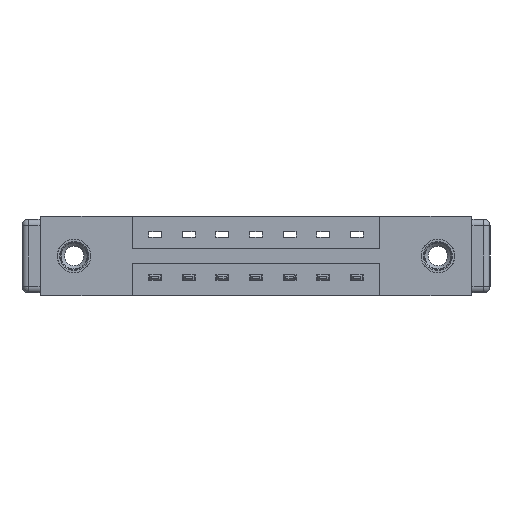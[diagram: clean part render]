
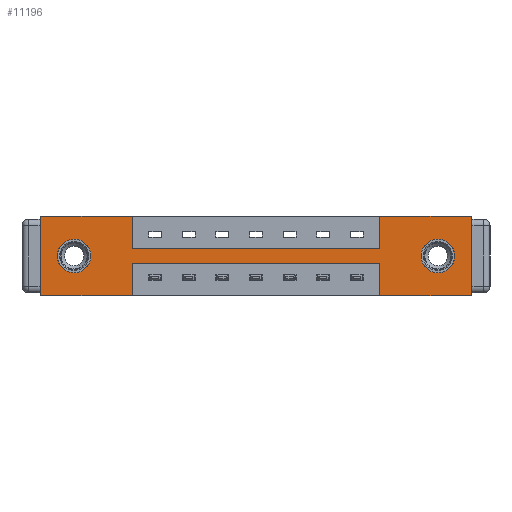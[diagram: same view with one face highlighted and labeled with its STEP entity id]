
A CAD part, front view. The second image highlights one B-rep face of the part: STEP entity #11196.
In plain terms, the highlighted planar face has unit normal (0, -1, 0).
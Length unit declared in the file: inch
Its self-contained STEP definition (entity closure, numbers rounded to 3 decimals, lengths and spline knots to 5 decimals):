
#67 = LINE ( 'NONE', #10866, #672 ) ;
#91 = EDGE_CURVE ( 'NONE', #1367, #12182, #2220, .T. ) ;
#122 = CARTESIAN_POINT ( 'NONE',  ( 0.425, 0., 0. ) ) ;
#201 = LINE ( 'NONE', #8902, #2409 ) ;
#452 = VECTOR ( 'NONE', #4776, 39.37008 ) ;
#585 = EDGE_LOOP ( 'NONE', ( #9365, #6233 ) ) ;
#595 = VERTEX_POINT ( 'NONE', #9121 ) ;
#672 = VECTOR ( 'NONE', #8072, 39.37008 ) ;
#810 = EDGE_CURVE ( 'NONE', #12182, #1367, #10688, .T. ) ;
#855 = ORIENTED_EDGE ( 'NONE', *, *, #3293, .F. ) ;
#969 = EDGE_CURVE ( 'NONE', #11671, #3734, #5891, .T. ) ;
#1114 = CARTESIAN_POINT ( 'NONE',  ( 0., 0., -0.37 ) ) ;
#1260 = CARTESIAN_POINT ( 'NONE',  ( 0., 0., -0.37 ) ) ;
#1367 = VERTEX_POINT ( 'NONE', #10426 ) ;
#1386 = LINE ( 'NONE', #1260, #7790 ) ;
#1478 = LINE ( 'NONE', #8052, #5311 ) ;
#1542 = AXIS2_PLACEMENT_3D ( 'NONE', #10679, #2914, #8666 ) ;
#1569 = VERTEX_POINT ( 'NONE', #11350 ) ;
#1675 = CARTESIAN_POINT ( 'NONE',  ( 0.425, 0., -0.15 ) ) ;
#1764 = CARTESIAN_POINT ( 'NONE',  ( 0.425, 0., -0.22 ) ) ;
#1878 = ORIENTED_EDGE ( 'NONE', *, *, #9618, .F. ) ;
#1949 = VECTOR ( 'NONE', #7408, 39.37008 ) ;
#2204 = CIRCLE ( 'NONE', #6351, 0.078 ) ;
#2214 = VECTOR ( 'NONE', #3540, 39.37008 ) ;
#2220 = CIRCLE ( 'NONE', #11262, 0.078 ) ;
#2244 = CARTESIAN_POINT ( 'NONE',  ( 1.843, 0., -0.185 ) ) ;
#2322 = CARTESIAN_POINT ( 'NONE',  ( 1.843, 0., -0.185 ) ) ;
#2409 = VECTOR ( 'NONE', #6393, 39.37008 ) ;
#2914 = DIRECTION ( 'NONE',  ( 0., 1., 0. ) ) ;
#3177 = ORIENTED_EDGE ( 'NONE', *, *, #4424, .T. ) ;
#3228 = DIRECTION ( 'NONE',  ( 0., 1., 0. ) ) ;
#3293 = EDGE_CURVE ( 'NONE', #7916, #9405, #5534, .T. ) ;
#3355 = CARTESIAN_POINT ( 'NONE',  ( 0.425, 0., -0.15 ) ) ;
#3430 = ORIENTED_EDGE ( 'NONE', *, *, #3432, .F. ) ;
#3432 = EDGE_CURVE ( 'NONE', #12314, #11671, #67, .T. ) ;
#3437 = EDGE_LOOP ( 'NONE', ( #6047, #3430, #1878, #6123, #7383, #6937, #9021, #7104, #6111, #855, #9856, #11272 ) ) ;
#3540 = DIRECTION ( 'NONE',  ( 0., 0., -1. ) ) ;
#3650 = CARTESIAN_POINT ( 'NONE',  ( 1.843, 0., -0.263 ) ) ;
#3734 = VERTEX_POINT ( 'NONE', #6125 ) ;
#3785 = AXIS2_PLACEMENT_3D ( 'NONE', #8471, #11432, #6671 ) ;
#3969 = DIRECTION ( 'NONE',  ( 0., 1., 0. ) ) ;
#4102 = CARTESIAN_POINT ( 'NONE',  ( 0.155, 0., -0.185 ) ) ;
#4159 = EDGE_CURVE ( 'NONE', #3734, #11264, #1386, .T. ) ;
#4201 = EDGE_CURVE ( 'NONE', #7337, #9529, #10927, .T. ) ;
#4424 = EDGE_CURVE ( 'NONE', #5752, #9320, #11345, .T. ) ;
#4460 = EDGE_CURVE ( 'NONE', #9405, #7337, #5518, .T. ) ;
#4485 = DIRECTION ( 'NONE',  ( 0., 0., -1. ) ) ;
#4542 = EDGE_LOOP ( 'NONE', ( #3177, #9253 ) ) ;
#4626 = VECTOR ( 'NONE', #12281, 39.37008 ) ;
#4670 = CARTESIAN_POINT ( 'NONE',  ( 1.573, 0., -0.37 ) ) ;
#4697 = CARTESIAN_POINT ( 'NONE',  ( 1.573, 0., 0. ) ) ;
#4776 = DIRECTION ( 'NONE',  ( 1., 0., 0. ) ) ;
#4903 = VECTOR ( 'NONE', #7796, 39.37008 ) ;
#5211 = DIRECTION ( 'NONE',  ( 0., 0., 1. ) ) ;
#5311 = VECTOR ( 'NONE', #5211, 39.37008 ) ;
#5518 = LINE ( 'NONE', #6795, #10326 ) ;
#5534 = LINE ( 'NONE', #9339, #4626 ) ;
#5566 = EDGE_CURVE ( 'NONE', #9529, #9190, #10666, .T. ) ;
#5608 = LINE ( 'NONE', #10615, #452 ) ;
#5752 = VERTEX_POINT ( 'NONE', #6143 ) ;
#5885 = DIRECTION ( 'NONE',  ( -1., 0., 0. ) ) ;
#5891 = LINE ( 'NONE', #10244, #7719 ) ;
#6019 = DIRECTION ( 'NONE',  ( 0., 0., 1. ) ) ;
#6047 = ORIENTED_EDGE ( 'NONE', *, *, #969, .F. ) ;
#6055 = DIRECTION ( 'NONE',  ( 0., 0., -1. ) ) ;
#6085 = DIRECTION ( 'NONE',  ( 0., 0., -1. ) ) ;
#6111 = ORIENTED_EDGE ( 'NONE', *, *, #4460, .F. ) ;
#6123 = ORIENTED_EDGE ( 'NONE', *, *, #7729, .F. ) ;
#6125 = CARTESIAN_POINT ( 'NONE',  ( 0.425, 0., -0.37 ) ) ;
#6143 = CARTESIAN_POINT ( 'NONE',  ( 1.843, 0., -0.107 ) ) ;
#6233 = ORIENTED_EDGE ( 'NONE', *, *, #810, .T. ) ;
#6351 = AXIS2_PLACEMENT_3D ( 'NONE', #2244, #3228, #6055 ) ;
#6393 = DIRECTION ( 'NONE',  ( -1., 0., 0. ) ) ;
#6636 = FACE_OUTER_BOUND ( 'NONE', #3437, .T. ) ;
#6671 = DIRECTION ( 'NONE',  ( 0., 0., -1. ) ) ;
#6795 = CARTESIAN_POINT ( 'NONE',  ( 0.425, 0., 0. ) ) ;
#6877 = LINE ( 'NONE', #10425, #1949 ) ;
#6937 = ORIENTED_EDGE ( 'NONE', *, *, #10081, .F. ) ;
#7065 = AXIS2_PLACEMENT_3D ( 'NONE', #2322, #10871, #6085 ) ;
#7104 = ORIENTED_EDGE ( 'NONE', *, *, #4201, .F. ) ;
#7236 = FACE_BOUND ( 'NONE', #585, .T. ) ;
#7265 = LINE ( 'NONE', #7524, #2214 ) ;
#7337 = VERTEX_POINT ( 'NONE', #1675 ) ;
#7383 = ORIENTED_EDGE ( 'NONE', *, *, #9859, .F. ) ;
#7403 = EDGE_CURVE ( 'NONE', #11264, #7916, #6877, .T. ) ;
#7407 = VERTEX_POINT ( 'NONE', #4670 ) ;
#7408 = DIRECTION ( 'NONE',  ( 0., 0., 1. ) ) ;
#7478 = PLANE ( 'NONE',  #3785 ) ;
#7524 = CARTESIAN_POINT ( 'NONE',  ( 1.998, 0., 0. ) ) ;
#7719 = VECTOR ( 'NONE', #4485, 39.37008 ) ;
#7729 = EDGE_CURVE ( 'NONE', #595, #7407, #201, .T. ) ;
#7790 = VECTOR ( 'NONE', #5885, 39.37008 ) ;
#7796 = DIRECTION ( 'NONE',  ( 1., 0., 0. ) ) ;
#7916 = VERTEX_POINT ( 'NONE', #10292 ) ;
#8052 = CARTESIAN_POINT ( 'NONE',  ( 1.573, 0., -0.37 ) ) ;
#8072 = DIRECTION ( 'NONE',  ( -1., 0., 0. ) ) ;
#8147 = VECTOR ( 'NONE', #11400, 39.37008 ) ;
#8274 = CARTESIAN_POINT ( 'NONE',  ( 1.573, 0., 0. ) ) ;
#8471 = CARTESIAN_POINT ( 'NONE',  ( 0., 0., -0.37 ) ) ;
#8666 = DIRECTION ( 'NONE',  ( 0., 0., 1. ) ) ;
#8902 = CARTESIAN_POINT ( 'NONE',  ( 0., 0., -0.37 ) ) ;
#9021 = ORIENTED_EDGE ( 'NONE', *, *, #5566, .F. ) ;
#9121 = CARTESIAN_POINT ( 'NONE',  ( 1.998, 0., -0.37 ) ) ;
#9146 = CARTESIAN_POINT ( 'NONE',  ( 1.573, 0., -0.22 ) ) ;
#9190 = VERTEX_POINT ( 'NONE', #8274 ) ;
#9253 = ORIENTED_EDGE ( 'NONE', *, *, #10735, .T. ) ;
#9320 = VERTEX_POINT ( 'NONE', #3650 ) ;
#9339 = CARTESIAN_POINT ( 'NONE',  ( 0., 0., 0. ) ) ;
#9363 = FACE_BOUND ( 'NONE', #4542, .T. ) ;
#9365 = ORIENTED_EDGE ( 'NONE', *, *, #91, .T. ) ;
#9405 = VERTEX_POINT ( 'NONE', #122 ) ;
#9529 = VERTEX_POINT ( 'NONE', #9620 ) ;
#9618 = EDGE_CURVE ( 'NONE', #7407, #12314, #1478, .T. ) ;
#9620 = CARTESIAN_POINT ( 'NONE',  ( 1.573, 0., -0.15 ) ) ;
#9856 = ORIENTED_EDGE ( 'NONE', *, *, #7403, .F. ) ;
#9859 = EDGE_CURVE ( 'NONE', #1569, #595, #7265, .T. ) ;
#10081 = EDGE_CURVE ( 'NONE', #9190, #1569, #5608, .T. ) ;
#10244 = CARTESIAN_POINT ( 'NONE',  ( 0.425, 0., -0.37 ) ) ;
#10292 = CARTESIAN_POINT ( 'NONE',  ( 0., 0., 0. ) ) ;
#10326 = VECTOR ( 'NONE', #11627, 39.37008 ) ;
#10425 = CARTESIAN_POINT ( 'NONE',  ( 0., 0., 0. ) ) ;
#10426 = CARTESIAN_POINT ( 'NONE',  ( 0.155, 0., -0.107 ) ) ;
#10615 = CARTESIAN_POINT ( 'NONE',  ( 0., 0., 0. ) ) ;
#10666 = LINE ( 'NONE', #4697, #8147 ) ;
#10679 = CARTESIAN_POINT ( 'NONE',  ( 0.155, 0., -0.185 ) ) ;
#10688 = CIRCLE ( 'NONE', #1542, 0.078 ) ;
#10735 = EDGE_CURVE ( 'NONE', #9320, #5752, #2204, .T. ) ;
#10866 = CARTESIAN_POINT ( 'NONE',  ( 0.425, 0., -0.22 ) ) ;
#10871 = DIRECTION ( 'NONE',  ( 0., 1., 0. ) ) ;
#10927 = LINE ( 'NONE', #3355, #4903 ) ;
#10932 = CARTESIAN_POINT ( 'NONE',  ( 0.155, 0., -0.263 ) ) ;
#11196 = ADVANCED_FACE ( 'NONE', ( #9363, #7236, #6636 ), #7478, .T. ) ;
#11262 = AXIS2_PLACEMENT_3D ( 'NONE', #4102, #3969, #6019 ) ;
#11264 = VERTEX_POINT ( 'NONE', #1114 ) ;
#11272 = ORIENTED_EDGE ( 'NONE', *, *, #4159, .F. ) ;
#11345 = CIRCLE ( 'NONE', #7065, 0.078 ) ;
#11350 = CARTESIAN_POINT ( 'NONE',  ( 1.998, 0., 0. ) ) ;
#11400 = DIRECTION ( 'NONE',  ( 0., 0., 1. ) ) ;
#11432 = DIRECTION ( 'NONE',  ( 0., -1., 0. ) ) ;
#11627 = DIRECTION ( 'NONE',  ( 0., 0., -1. ) ) ;
#11671 = VERTEX_POINT ( 'NONE', #1764 ) ;
#12182 = VERTEX_POINT ( 'NONE', #10932 ) ;
#12281 = DIRECTION ( 'NONE',  ( 1., 0., 0. ) ) ;
#12314 = VERTEX_POINT ( 'NONE', #9146 ) ;
